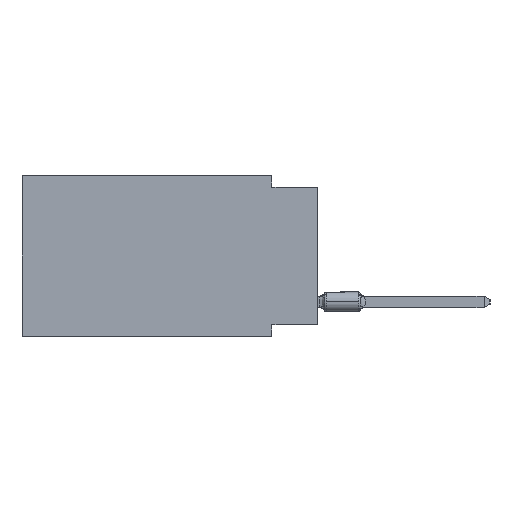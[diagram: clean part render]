
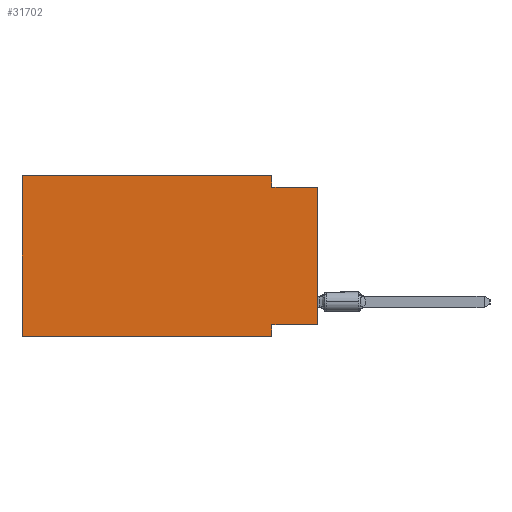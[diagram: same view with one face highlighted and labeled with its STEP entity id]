
A CAD part, left-side view. The second image highlights one B-rep face of the part: STEP entity #31702.
In plain terms, the highlighted planar face has unit normal (-1, 0, 0).
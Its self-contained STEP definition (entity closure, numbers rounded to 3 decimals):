
#171 = VERTEX_POINT ( 'NONE', #9678 ) ;
#310 = EDGE_CURVE ( 'NONE', #1983, #47865, #57449, .T. ) ;
#1983 = VERTEX_POINT ( 'NONE', #6738 ) ;
#3043 = CARTESIAN_POINT ( 'NONE',  ( 0., 0., -0.635 ) ) ;
#3087 = ORIENTED_EDGE ( 'NONE', *, *, #11459, .F. ) ;
#3418 = PLANE ( 'NONE',  #43479 ) ;
#3705 = LINE ( 'NONE', #11622, #27545 ) ;
#5305 = VERTEX_POINT ( 'NONE', #32669 ) ;
#5387 = VECTOR ( 'NONE', #16892, 1000. ) ;
#6037 = CARTESIAN_POINT ( 'NONE',  ( 0., 0., -0.635 ) ) ;
#6329 = CARTESIAN_POINT ( 'NONE',  ( 0., 16.383, 0. ) ) ;
#6738 = CARTESIAN_POINT ( 'NONE',  ( 0., 16.383, -8.89 ) ) ;
#8574 = CARTESIAN_POINT ( 'NONE',  ( 0., 16.383, 0. ) ) ;
#9553 = CARTESIAN_POINT ( 'NONE',  ( 0., 16.383, 0. ) ) ;
#9678 = CARTESIAN_POINT ( 'NONE',  ( 0., 0., -8.255 ) ) ;
#11459 = EDGE_CURVE ( 'NONE', #171, #35912, #57204, .T. ) ;
#11622 = CARTESIAN_POINT ( 'NONE',  ( 0., 0., 0. ) ) ;
#13796 = ORIENTED_EDGE ( 'NONE', *, *, #310, .T. ) ;
#14953 = ORIENTED_EDGE ( 'NONE', *, *, #49834, .F. ) ;
#15655 = ORIENTED_EDGE ( 'NONE', *, *, #23488, .F. ) ;
#15736 = DIRECTION ( 'NONE',  ( 0., -1., 0. ) ) ;
#16035 = LINE ( 'NONE', #6329, #51050 ) ;
#16892 = DIRECTION ( 'NONE',  ( 0., -1., 0. ) ) ;
#17204 = CARTESIAN_POINT ( 'NONE',  ( 0., 2.54, 0. ) ) ;
#17678 = DIRECTION ( 'NONE',  ( 1., 0., 0. ) ) ;
#17833 = VERTEX_POINT ( 'NONE', #44088 ) ;
#21860 = ORIENTED_EDGE ( 'NONE', *, *, #30242, .F. ) ;
#22224 = FACE_OUTER_BOUND ( 'NONE', #45136, .T. ) ;
#23488 = EDGE_CURVE ( 'NONE', #35912, #47865, #27272, .T. ) ;
#25484 = LINE ( 'NONE', #3043, #52786 ) ;
#25688 = DIRECTION ( 'NONE',  ( 0., 0., -1. ) ) ;
#26667 = LINE ( 'NONE', #54508, #37343 ) ;
#27272 = LINE ( 'NONE', #50554, #59220 ) ;
#27545 = VECTOR ( 'NONE', #44596, 1000. ) ;
#27568 = DIRECTION ( 'NONE',  ( 0., 0., -1. ) ) ;
#27984 = EDGE_CURVE ( 'NONE', #55142, #17833, #16035, .T. ) ;
#29669 = DIRECTION ( 'NONE',  ( 0., 1., 0. ) ) ;
#30242 = EDGE_CURVE ( 'NONE', #17833, #5305, #48391, .T. ) ;
#31702 = ADVANCED_FACE ( 'NONE', ( #22224 ), #3418, .F. ) ;
#32669 = CARTESIAN_POINT ( 'NONE',  ( 0., 2.54, -0.635 ) ) ;
#34865 = DIRECTION ( 'NONE',  ( 0., -1., 0. ) ) ;
#35912 = VERTEX_POINT ( 'NONE', #50344 ) ;
#37343 = VECTOR ( 'NONE', #48478, 1000. ) ;
#38250 = ORIENTED_EDGE ( 'NONE', *, *, #48152, .T. ) ;
#39262 = VERTEX_POINT ( 'NONE', #6037 ) ;
#43479 = AXIS2_PLACEMENT_3D ( 'NONE', #8574, #17678, #49737 ) ;
#44088 = CARTESIAN_POINT ( 'NONE',  ( 0., 2.54, 0. ) ) ;
#44596 = DIRECTION ( 'NONE',  ( 0., 0., 1. ) ) ;
#44847 = VECTOR ( 'NONE', #29669, 1000. ) ;
#45136 = EDGE_LOOP ( 'NONE', ( #38250, #53054, #21860, #54978, #14953, #13796, #15655, #3087 ) ) ;
#47865 = VERTEX_POINT ( 'NONE', #50987 ) ;
#48152 = EDGE_CURVE ( 'NONE', #171, #39262, #3705, .T. ) ;
#48391 = LINE ( 'NONE', #17204, #52217 ) ;
#48478 = DIRECTION ( 'NONE',  ( 0., 0., 1. ) ) ;
#49257 = CARTESIAN_POINT ( 'NONE',  ( 0., 16.383, -8.89 ) ) ;
#49737 = DIRECTION ( 'NONE',  ( 0., 0., -1. ) ) ;
#49834 = EDGE_CURVE ( 'NONE', #1983, #55142, #26667, .T. ) ;
#49866 = EDGE_CURVE ( 'NONE', #5305, #39262, #25484, .T. ) ;
#50344 = CARTESIAN_POINT ( 'NONE',  ( 0., 2.54, -8.255 ) ) ;
#50554 = CARTESIAN_POINT ( 'NONE',  ( 0., 2.54, -8.89 ) ) ;
#50987 = CARTESIAN_POINT ( 'NONE',  ( 0., 2.54, -8.89 ) ) ;
#51050 = VECTOR ( 'NONE', #15736, 1000. ) ;
#52217 = VECTOR ( 'NONE', #25688, 1000. ) ;
#52663 = CARTESIAN_POINT ( 'NONE',  ( 0., 0., -8.255 ) ) ;
#52786 = VECTOR ( 'NONE', #34865, 1000. ) ;
#53054 = ORIENTED_EDGE ( 'NONE', *, *, #49866, .F. ) ;
#54508 = CARTESIAN_POINT ( 'NONE',  ( 0., 16.383, 0. ) ) ;
#54978 = ORIENTED_EDGE ( 'NONE', *, *, #27984, .F. ) ;
#55142 = VERTEX_POINT ( 'NONE', #9553 ) ;
#57204 = LINE ( 'NONE', #52663, #44847 ) ;
#57449 = LINE ( 'NONE', #49257, #5387 ) ;
#59220 = VECTOR ( 'NONE', #27568, 1000. ) ;
